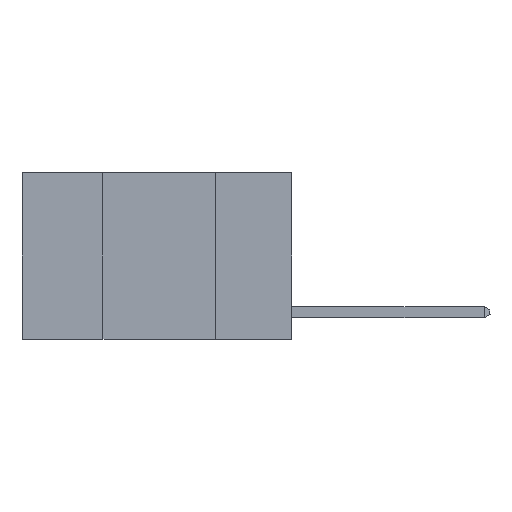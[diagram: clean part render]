
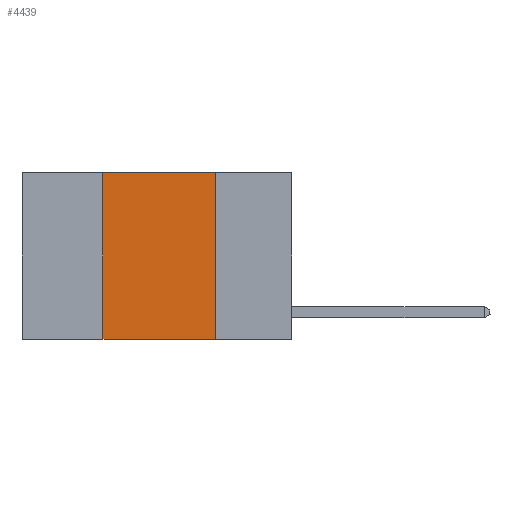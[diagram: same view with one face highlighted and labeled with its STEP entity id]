
A CAD part, left-side view. The second image highlights one B-rep face of the part: STEP entity #4439.
In plain terms, the highlighted planar face has unit normal (-1, 0, 0).
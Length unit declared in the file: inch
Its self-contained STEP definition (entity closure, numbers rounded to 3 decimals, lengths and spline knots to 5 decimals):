
#689 = DIRECTION ( 'NONE',  ( 1., 0., 0. ) ) ;
#1857 = VECTOR ( 'NONE', #17476, 39.37008 ) ;
#3123 = AXIS2_PLACEMENT_3D ( 'NONE', #5911, #689, #13085 ) ;
#3392 = DIRECTION ( 'NONE',  ( 0., 0., 1. ) ) ;
#4140 = PLANE ( 'NONE',  #3123 ) ;
#4201 = ORIENTED_EDGE ( 'NONE', *, *, #5280, .F. ) ;
#4439 = ADVANCED_FACE ( 'NONE', ( #11888 ), #4140, .F. ) ;
#4735 = VECTOR ( 'NONE', #3392, 39.37008 ) ;
#4752 = EDGE_CURVE ( 'NONE', #22361, #10640, #5722, .T. ) ;
#5169 = VECTOR ( 'NONE', #10536, 39.37008 ) ;
#5280 = EDGE_CURVE ( 'NONE', #15122, #10640, #6524, .T. ) ;
#5722 = LINE ( 'NONE', #17819, #5169 ) ;
#5882 = CARTESIAN_POINT ( 'NONE',  ( 0., 0.42, -0.37 ) ) ;
#5911 = CARTESIAN_POINT ( 'NONE',  ( 0., 0.6, 0. ) ) ;
#6243 = VECTOR ( 'NONE', #21787, 39.37008 ) ;
#6524 = LINE ( 'NONE', #12051, #1857 ) ;
#7913 = EDGE_CURVE ( 'NONE', #22361, #9015, #19004, .T. ) ;
#8039 = CARTESIAN_POINT ( 'NONE',  ( 0., 0.17, 0. ) ) ;
#9015 = VERTEX_POINT ( 'NONE', #19022 ) ;
#10494 = ORIENTED_EDGE ( 'NONE', *, *, #4752, .T. ) ;
#10536 = DIRECTION ( 'NONE',  ( 0., -1., 0. ) ) ;
#10640 = VERTEX_POINT ( 'NONE', #18570 ) ;
#11888 = FACE_OUTER_BOUND ( 'NONE', #16481, .T. ) ;
#12051 = CARTESIAN_POINT ( 'NONE',  ( 0., 0.17, 0. ) ) ;
#13085 = DIRECTION ( 'NONE',  ( 0., 0., -1. ) ) ;
#15122 = VERTEX_POINT ( 'NONE', #8039 ) ;
#15602 = ORIENTED_EDGE ( 'NONE', *, *, #19351, .F. ) ;
#16481 = EDGE_LOOP ( 'NONE', ( #4201, #15602, #19284, #10494 ) ) ;
#17476 = DIRECTION ( 'NONE',  ( 0., 0., -1. ) ) ;
#17819 = CARTESIAN_POINT ( 'NONE',  ( 0., 0.6, -0.37 ) ) ;
#18570 = CARTESIAN_POINT ( 'NONE',  ( 0., 0.17, -0.37 ) ) ;
#19004 = LINE ( 'NONE', #22998, #4735 ) ;
#19022 = CARTESIAN_POINT ( 'NONE',  ( 0., 0.42, 0. ) ) ;
#19284 = ORIENTED_EDGE ( 'NONE', *, *, #7913, .F. ) ;
#19351 = EDGE_CURVE ( 'NONE', #9015, #15122, #20525, .T. ) ;
#20018 = CARTESIAN_POINT ( 'NONE',  ( 0., 0.6, 0. ) ) ;
#20525 = LINE ( 'NONE', #20018, #6243 ) ;
#21787 = DIRECTION ( 'NONE',  ( 0., -1., 0. ) ) ;
#22361 = VERTEX_POINT ( 'NONE', #5882 ) ;
#22998 = CARTESIAN_POINT ( 'NONE',  ( 0., 0.42, 0. ) ) ;
